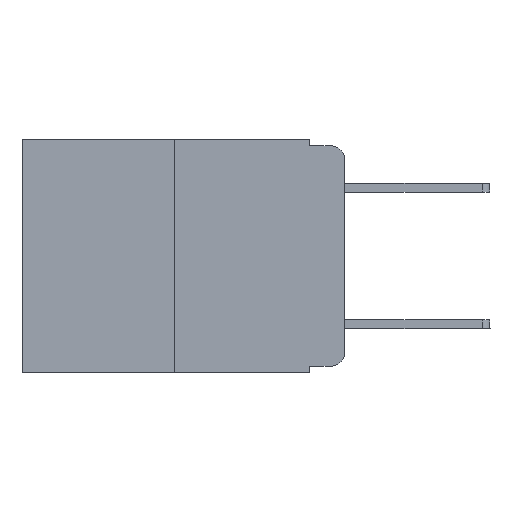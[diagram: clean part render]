
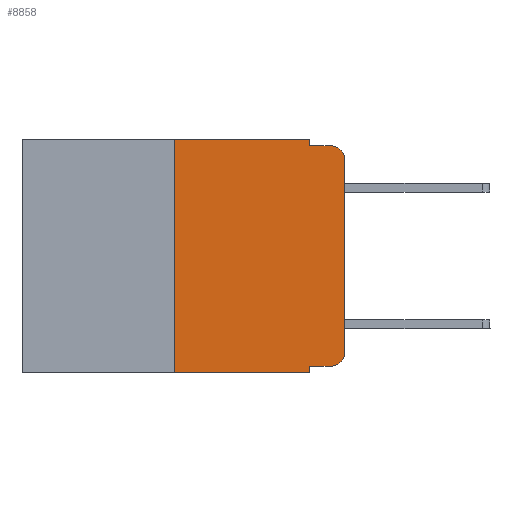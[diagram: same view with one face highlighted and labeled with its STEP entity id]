
A CAD part, left-side view. The second image highlights one B-rep face of the part: STEP entity #8858.
In plain terms, the highlighted planar face has unit normal (-1, 0, 0).
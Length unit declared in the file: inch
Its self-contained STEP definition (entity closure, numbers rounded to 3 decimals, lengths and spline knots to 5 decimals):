
#96 = VECTOR ( 'NONE', #22979, 39.37008 ) ;
#191 = VECTOR ( 'NONE', #21636, 39.37008 ) ;
#210 = LINE ( 'NONE', #14217, #15443 ) ;
#675 = DIRECTION ( 'NONE',  ( 0., -1., 0. ) ) ;
#1158 = EDGE_CURVE ( 'NONE', #14622, #8579, #11118, .T. ) ;
#1379 = EDGE_CURVE ( 'NONE', #5180, #12701, #4315, .T. ) ;
#1832 = CARTESIAN_POINT ( 'NONE',  ( 0., 0.473, -0.343 ) ) ;
#2075 = LINE ( 'NONE', #1832, #12115 ) ;
#2226 = DIRECTION ( 'NONE',  ( 0., 0., -1. ) ) ;
#2340 = VERTEX_POINT ( 'NONE', #5029 ) ;
#2424 = CARTESIAN_POINT ( 'NONE',  ( 0., 0.473, 0. ) ) ;
#3256 = ORIENTED_EDGE ( 'NONE', *, *, #24872, .T. ) ;
#4052 = CIRCLE ( 'NONE', #18667, 0.02 ) ;
#4315 = LINE ( 'NONE', #12334, #10301 ) ;
#4911 = ORIENTED_EDGE ( 'NONE', *, *, #15210, .F. ) ;
#5029 = CARTESIAN_POINT ( 'NONE',  ( 0., 0.051, -0.343 ) ) ;
#5180 = VERTEX_POINT ( 'NONE', #16711 ) ;
#5194 = ORIENTED_EDGE ( 'NONE', *, *, #1158, .T. ) ;
#5217 = EDGE_CURVE ( 'NONE', #8579, #21671, #25176, .T. ) ;
#5738 = FACE_OUTER_BOUND ( 'NONE', #17250, .T. ) ;
#5883 = DIRECTION ( 'NONE',  ( 0., -1., 0. ) ) ;
#6365 = DIRECTION ( 'NONE',  ( 0., 0., -1. ) ) ;
#6419 = ORIENTED_EDGE ( 'NONE', *, *, #21719, .T. ) ;
#6546 = CARTESIAN_POINT ( 'NONE',  ( 0., 0., -0.313 ) ) ;
#6743 = VERTEX_POINT ( 'NONE', #22026 ) ;
#7557 = LINE ( 'NONE', #17357, #14914 ) ;
#7627 = VECTOR ( 'NONE', #675, 39.37008 ) ;
#8053 = EDGE_CURVE ( 'NONE', #17218, #2340, #7557, .T. ) ;
#8102 = DIRECTION ( 'NONE',  ( 0., 0., -1. ) ) ;
#8235 = DIRECTION ( 'NONE',  ( -1., 0., 0. ) ) ;
#8579 = VERTEX_POINT ( 'NONE', #6546 ) ;
#8716 = CARTESIAN_POINT ( 'NONE',  ( 0., 0.051, -0.333 ) ) ;
#8858 = ADVANCED_FACE ( 'NONE', ( #5738 ), #19613, .F. ) ;
#10301 = VECTOR ( 'NONE', #20277, 39.37008 ) ;
#10986 = CARTESIAN_POINT ( 'NONE',  ( 0., 0.051, 0. ) ) ;
#11118 = CIRCLE ( 'NONE', #17784, 0.02 ) ;
#11150 = CARTESIAN_POINT ( 'NONE',  ( 0., 0.25, -0.343 ) ) ;
#11399 = LINE ( 'NONE', #15191, #23482 ) ;
#11475 = CARTESIAN_POINT ( 'NONE',  ( 0., 0., 0. ) ) ;
#11833 = ORIENTED_EDGE ( 'NONE', *, *, #15437, .F. ) ;
#11950 = CARTESIAN_POINT ( 'NONE',  ( 0., 0.02, -0.313 ) ) ;
#12115 = VECTOR ( 'NONE', #5883, 39.37008 ) ;
#12334 = CARTESIAN_POINT ( 'NONE',  ( 0., 0.473, 0. ) ) ;
#12407 = ORIENTED_EDGE ( 'NONE', *, *, #8053, .F. ) ;
#12701 = VERTEX_POINT ( 'NONE', #24152 ) ;
#14217 = CARTESIAN_POINT ( 'NONE',  ( 0., 0.051, -0.333 ) ) ;
#14231 = DIRECTION ( 'NONE',  ( 1., 0., 0. ) ) ;
#14622 = VERTEX_POINT ( 'NONE', #18248 ) ;
#14914 = VECTOR ( 'NONE', #23613, 39.37008 ) ;
#15191 = CARTESIAN_POINT ( 'NONE',  ( 0., 0.25, 0. ) ) ;
#15210 = EDGE_CURVE ( 'NONE', #18289, #5180, #11399, .T. ) ;
#15437 = EDGE_CURVE ( 'NONE', #12701, #6743, #18648, .T. ) ;
#15443 = VECTOR ( 'NONE', #22171, 39.37008 ) ;
#15941 = CARTESIAN_POINT ( 'NONE',  ( 0., 0.02, -0.03 ) ) ;
#15977 = ORIENTED_EDGE ( 'NONE', *, *, #5217, .T. ) ;
#16337 = EDGE_CURVE ( 'NONE', #6743, #19901, #16803, .T. ) ;
#16344 = ORIENTED_EDGE ( 'NONE', *, *, #25212, .T. ) ;
#16537 = CARTESIAN_POINT ( 'NONE',  ( 0., 0.051, -0.01 ) ) ;
#16711 = CARTESIAN_POINT ( 'NONE',  ( 0., 0.25, 0. ) ) ;
#16803 = LINE ( 'NONE', #16537, #7627 ) ;
#17218 = VERTEX_POINT ( 'NONE', #8716 ) ;
#17250 = EDGE_LOOP ( 'NONE', ( #15977, #6419, #23983, #11833, #20438, #4911, #16344, #12407, #3256, #5194 ) ) ;
#17357 = CARTESIAN_POINT ( 'NONE',  ( 0., 0.051, 0. ) ) ;
#17784 = AXIS2_PLACEMENT_3D ( 'NONE', #11950, #17942, #2226 ) ;
#17942 = DIRECTION ( 'NONE',  ( -1., 0., 0. ) ) ;
#18248 = CARTESIAN_POINT ( 'NONE',  ( 0., 0.02, -0.333 ) ) ;
#18289 = VERTEX_POINT ( 'NONE', #11150 ) ;
#18648 = LINE ( 'NONE', #10986, #96 ) ;
#18667 = AXIS2_PLACEMENT_3D ( 'NONE', #15941, #8235, #8102 ) ;
#19466 = DIRECTION ( 'NONE',  ( 0., 0., 1. ) ) ;
#19613 = PLANE ( 'NONE',  #21600 ) ;
#19901 = VERTEX_POINT ( 'NONE', #20630 ) ;
#20277 = DIRECTION ( 'NONE',  ( 0., -1., 0. ) ) ;
#20438 = ORIENTED_EDGE ( 'NONE', *, *, #1379, .F. ) ;
#20484 = CARTESIAN_POINT ( 'NONE',  ( 0., 0., -0.03 ) ) ;
#20630 = CARTESIAN_POINT ( 'NONE',  ( 0., 0.02, -0.01 ) ) ;
#21600 = AXIS2_PLACEMENT_3D ( 'NONE', #2424, #14231, #6365 ) ;
#21636 = DIRECTION ( 'NONE',  ( 0., 0., 1. ) ) ;
#21671 = VERTEX_POINT ( 'NONE', #20484 ) ;
#21719 = EDGE_CURVE ( 'NONE', #21671, #19901, #4052, .T. ) ;
#22026 = CARTESIAN_POINT ( 'NONE',  ( 0., 0.051, -0.01 ) ) ;
#22171 = DIRECTION ( 'NONE',  ( 0., -1., 0. ) ) ;
#22979 = DIRECTION ( 'NONE',  ( 0., 0., -1. ) ) ;
#23482 = VECTOR ( 'NONE', #19466, 39.37008 ) ;
#23613 = DIRECTION ( 'NONE',  ( 0., 0., -1. ) ) ;
#23983 = ORIENTED_EDGE ( 'NONE', *, *, #16337, .F. ) ;
#24152 = CARTESIAN_POINT ( 'NONE',  ( 0., 0.051, 0. ) ) ;
#24872 = EDGE_CURVE ( 'NONE', #17218, #14622, #210, .T. ) ;
#25176 = LINE ( 'NONE', #11475, #191 ) ;
#25212 = EDGE_CURVE ( 'NONE', #18289, #2340, #2075, .T. ) ;
